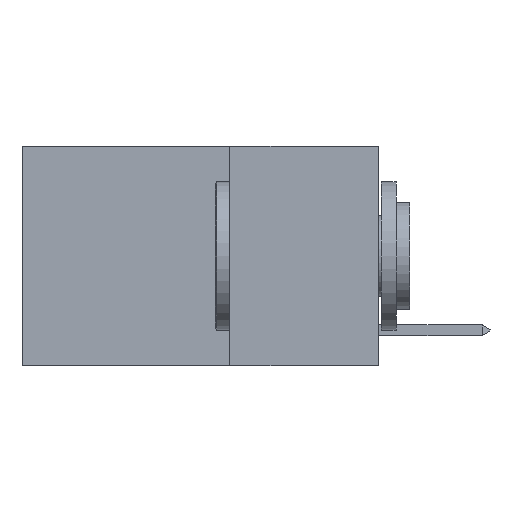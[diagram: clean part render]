
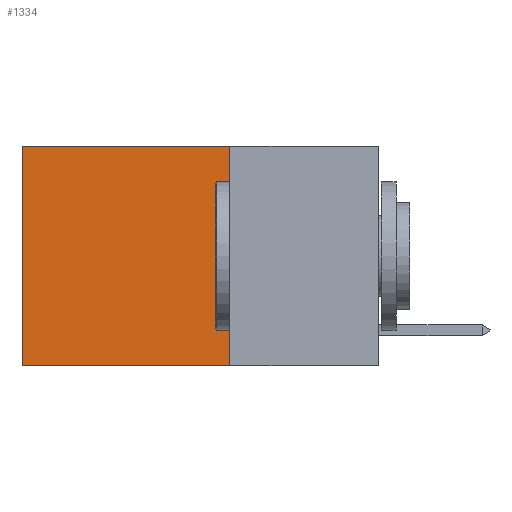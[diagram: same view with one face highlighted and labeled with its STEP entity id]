
A CAD part, left-side view. The second image highlights one B-rep face of the part: STEP entity #1334.
In plain terms, the highlighted planar face has unit normal (-1, 0, 0).
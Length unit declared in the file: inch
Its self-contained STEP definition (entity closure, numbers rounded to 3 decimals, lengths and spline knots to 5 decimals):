
#66 = VERTEX_POINT ( 'NONE', #336 ) ;
#336 = CARTESIAN_POINT ( 'NONE',  ( 0.2625, 0.6, 0. ) ) ;
#372 = ORIENTED_EDGE ( 'NONE', *, *, #4426, .T. ) ;
#544 = VECTOR ( 'NONE', #6972, 39.37008 ) ;
#944 = EDGE_CURVE ( 'NONE', #5393, #7784, #6519, .T. ) ;
#1334 = ADVANCED_FACE ( 'NONE', ( #13739 ), #10367, .F. ) ;
#2624 = CARTESIAN_POINT ( 'NONE',  ( 0.2625, 0.25, 0. ) ) ;
#2663 = DIRECTION ( 'NONE',  ( 0., 1., 0. ) ) ;
#3100 = DIRECTION ( 'NONE',  ( 0., 0., -1. ) ) ;
#3866 = CARTESIAN_POINT ( 'NONE',  ( 0.2625, 0.25, -0.37 ) ) ;
#3933 = AXIS2_PLACEMENT_3D ( 'NONE', #4771, #4546, #12724 ) ;
#4243 = ORIENTED_EDGE ( 'NONE', *, *, #944, .F. ) ;
#4426 = EDGE_CURVE ( 'NONE', #66, #7679, #13723, .T. ) ;
#4463 = DIRECTION ( 'NONE',  ( 0., 0., -1. ) ) ;
#4546 = DIRECTION ( 'NONE',  ( 1., 0., 0. ) ) ;
#4771 = CARTESIAN_POINT ( 'NONE',  ( 0.2625, 0.25, 0. ) ) ;
#5393 = VERTEX_POINT ( 'NONE', #2624 ) ;
#5585 = VECTOR ( 'NONE', #2663, 39.37008 ) ;
#6519 = LINE ( 'NONE', #8750, #7337 ) ;
#6972 = DIRECTION ( 'NONE',  ( 0., 1., 0. ) ) ;
#7337 = VECTOR ( 'NONE', #3100, 39.37008 ) ;
#7679 = VERTEX_POINT ( 'NONE', #11165 ) ;
#7784 = VERTEX_POINT ( 'NONE', #3866 ) ;
#7819 = ORIENTED_EDGE ( 'NONE', *, *, #9114, .T. ) ;
#8147 = CARTESIAN_POINT ( 'NONE',  ( 0.2625, 0.25, -0.37 ) ) ;
#8750 = CARTESIAN_POINT ( 'NONE',  ( 0.2625, 0.25, 0. ) ) ;
#9114 = EDGE_CURVE ( 'NONE', #5393, #66, #12267, .T. ) ;
#9343 = LINE ( 'NONE', #8147, #544 ) ;
#10342 = ORIENTED_EDGE ( 'NONE', *, *, #11856, .F. ) ;
#10367 = PLANE ( 'NONE',  #3933 ) ;
#11165 = CARTESIAN_POINT ( 'NONE',  ( 0.2625, 0.6, -0.37 ) ) ;
#11536 = VECTOR ( 'NONE', #4463, 39.37008 ) ;
#11856 = EDGE_CURVE ( 'NONE', #7784, #7679, #9343, .T. ) ;
#12267 = LINE ( 'NONE', #13360, #5585 ) ;
#12352 = EDGE_LOOP ( 'NONE', ( #372, #10342, #4243, #7819 ) ) ;
#12549 = CARTESIAN_POINT ( 'NONE',  ( 0.2625, 0.6, 0. ) ) ;
#12724 = DIRECTION ( 'NONE',  ( 0., 0., -1. ) ) ;
#13360 = CARTESIAN_POINT ( 'NONE',  ( 0.2625, 0.25, 0. ) ) ;
#13723 = LINE ( 'NONE', #12549, #11536 ) ;
#13739 = FACE_OUTER_BOUND ( 'NONE', #12352, .T. ) ;
